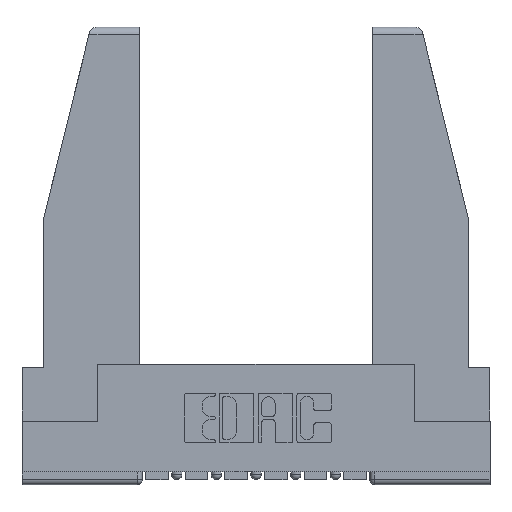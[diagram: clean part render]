
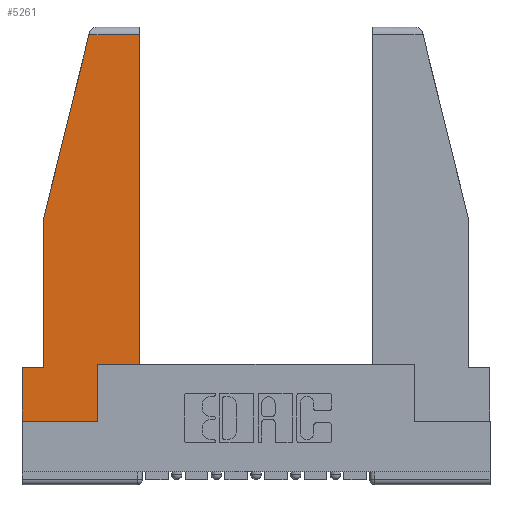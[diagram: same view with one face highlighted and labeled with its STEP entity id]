
A CAD part, top view. The second image highlights one B-rep face of the part: STEP entity #5261.
In plain terms, the highlighted planar face has unit normal (0, 0, 1).
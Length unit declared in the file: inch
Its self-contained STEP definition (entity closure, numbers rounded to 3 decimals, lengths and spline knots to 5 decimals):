
#73 = CARTESIAN_POINT ( 'NONE',  ( 0.461, 1.52, 0. ) ) ;
#416 = CARTESIAN_POINT ( 'NONE',  ( 0., 0., 0. ) ) ;
#540 = EDGE_LOOP ( 'NONE', ( #6961, #12281, #1165, #3344, #7194, #10170, #1992, #6315, #4431 ) ) ;
#910 = CARTESIAN_POINT ( 'NONE',  ( 0.271, 1.55, 0. ) ) ;
#1165 = ORIENTED_EDGE ( 'NONE', *, *, #9853, .T. ) ;
#1574 = CARTESIAN_POINT ( 'NONE',  ( 0., 0., 0. ) ) ;
#1669 = VECTOR ( 'NONE', #1719, 39.37008 ) ;
#1687 = LINE ( 'NONE', #3269, #12067 ) ;
#1719 = DIRECTION ( 'NONE',  ( -1., 0., 0. ) ) ;
#1840 = VERTEX_POINT ( 'NONE', #3769 ) ;
#1897 = VERTEX_POINT ( 'NONE', #6950 ) ;
#1911 = FACE_OUTER_BOUND ( 'NONE', #540, .T. ) ;
#1992 = ORIENTED_EDGE ( 'NONE', *, *, #10947, .T. ) ;
#2035 = PLANE ( 'NONE',  #11664 ) ;
#2053 = LINE ( 'NONE', #2567, #4275 ) ;
#2088 = VERTEX_POINT ( 'NONE', #10209 ) ;
#2297 = LINE ( 'NONE', #4643, #1669 ) ;
#2567 = CARTESIAN_POINT ( 'NONE',  ( 0.297, 0.223, 0. ) ) ;
#2610 = EDGE_CURVE ( 'NONE', #2088, #8212, #7209, .T. ) ;
#2855 = CARTESIAN_POINT ( 'NONE',  ( 0., 0.21, 0. ) ) ;
#2945 = VECTOR ( 'NONE', #11036, 39.37008 ) ;
#3020 = VERTEX_POINT ( 'NONE', #7892 ) ;
#3237 = CARTESIAN_POINT ( 'NONE',  ( 0.086, 0.8, 0. ) ) ;
#3269 = CARTESIAN_POINT ( 'NONE',  ( 0.297, 0., 0. ) ) ;
#3344 = ORIENTED_EDGE ( 'NONE', *, *, #6811, .T. ) ;
#3769 = CARTESIAN_POINT ( 'NONE',  ( 0.297, 0.223, 0. ) ) ;
#4275 = VECTOR ( 'NONE', #8486, 39.37008 ) ;
#4416 = DIRECTION ( 'NONE',  ( 1., 0., 0. ) ) ;
#4431 = ORIENTED_EDGE ( 'NONE', *, *, #5400, .T. ) ;
#4643 = CARTESIAN_POINT ( 'NONE',  ( 0., 1.52, 0. ) ) ;
#5122 = VERTEX_POINT ( 'NONE', #9862 ) ;
#5217 = LINE ( 'NONE', #416, #9155 ) ;
#5221 = DIRECTION ( 'NONE',  ( 1., 0., 0. ) ) ;
#5261 = ADVANCED_FACE ( 'NONE', ( #1911 ), #2035, .T. ) ;
#5400 = EDGE_CURVE ( 'NONE', #1840, #2088, #2053, .T. ) ;
#5664 = VECTOR ( 'NONE', #9062, 39.37008 ) ;
#5799 = VECTOR ( 'NONE', #12967, 39.37008 ) ;
#6046 = VECTOR ( 'NONE', #7866, 39.37008 ) ;
#6315 = ORIENTED_EDGE ( 'NONE', *, *, #7002, .T. ) ;
#6404 = EDGE_CURVE ( 'NONE', #10200, #5122, #8803, .T. ) ;
#6811 = EDGE_CURVE ( 'NONE', #7571, #10200, #12850, .T. ) ;
#6950 = CARTESIAN_POINT ( 'NONE',  ( 0.297, 0., 0. ) ) ;
#6961 = ORIENTED_EDGE ( 'NONE', *, *, #2610, .T. ) ;
#6995 = DIRECTION ( 'NONE',  ( 0., 0., 1. ) ) ;
#7002 = EDGE_CURVE ( 'NONE', #1897, #1840, #1687, .T. ) ;
#7194 = ORIENTED_EDGE ( 'NONE', *, *, #6404, .T. ) ;
#7209 = LINE ( 'NONE', #12960, #2945 ) ;
#7571 = VERTEX_POINT ( 'NONE', #3237 ) ;
#7692 = CARTESIAN_POINT ( 'NONE',  ( 0.086, 0.8, 0. ) ) ;
#7866 = DIRECTION ( 'NONE',  ( -0.239, -0.971, 0. ) ) ;
#7892 = CARTESIAN_POINT ( 'NONE',  ( 0.2636, 1.52, 0. ) ) ;
#8212 = VERTEX_POINT ( 'NONE', #73 ) ;
#8336 = VECTOR ( 'NONE', #11715, 39.37008 ) ;
#8418 = LINE ( 'NONE', #910, #6046 ) ;
#8486 = DIRECTION ( 'NONE',  ( 1., 0., 0. ) ) ;
#8500 = EDGE_CURVE ( 'NONE', #8212, #3020, #2297, .T. ) ;
#8803 = LINE ( 'NONE', #2855, #5664 ) ;
#8984 = VERTEX_POINT ( 'NONE', #1574 ) ;
#9062 = DIRECTION ( 'NONE',  ( -1., 0., 0. ) ) ;
#9093 = CARTESIAN_POINT ( 'NONE',  ( 0., 0., 0. ) ) ;
#9155 = VECTOR ( 'NONE', #4416, 39.37008 ) ;
#9853 = EDGE_CURVE ( 'NONE', #3020, #7571, #8418, .T. ) ;
#9862 = CARTESIAN_POINT ( 'NONE',  ( 0., 0.21, 0. ) ) ;
#10067 = CARTESIAN_POINT ( 'NONE',  ( 0., 0.21, 0. ) ) ;
#10170 = ORIENTED_EDGE ( 'NONE', *, *, #12612, .T. ) ;
#10200 = VERTEX_POINT ( 'NONE', #11523 ) ;
#10209 = CARTESIAN_POINT ( 'NONE',  ( 0.461, 0.223, 0. ) ) ;
#10303 = DIRECTION ( 'NONE',  ( 0., 1., 0. ) ) ;
#10947 = EDGE_CURVE ( 'NONE', #8984, #1897, #5217, .T. ) ;
#11036 = DIRECTION ( 'NONE',  ( 0., 1., 0. ) ) ;
#11523 = CARTESIAN_POINT ( 'NONE',  ( 0.086, 0.21, 0. ) ) ;
#11664 = AXIS2_PLACEMENT_3D ( 'NONE', #9093, #6995, #5221 ) ;
#11715 = DIRECTION ( 'NONE',  ( 0., -1., 0. ) ) ;
#12067 = VECTOR ( 'NONE', #10303, 39.37008 ) ;
#12281 = ORIENTED_EDGE ( 'NONE', *, *, #8500, .T. ) ;
#12385 = LINE ( 'NONE', #10067, #5799 ) ;
#12612 = EDGE_CURVE ( 'NONE', #5122, #8984, #12385, .T. ) ;
#12850 = LINE ( 'NONE', #7692, #8336 ) ;
#12960 = CARTESIAN_POINT ( 'NONE',  ( 0.461, 0.223, 0. ) ) ;
#12967 = DIRECTION ( 'NONE',  ( 0., -1., 0. ) ) ;
